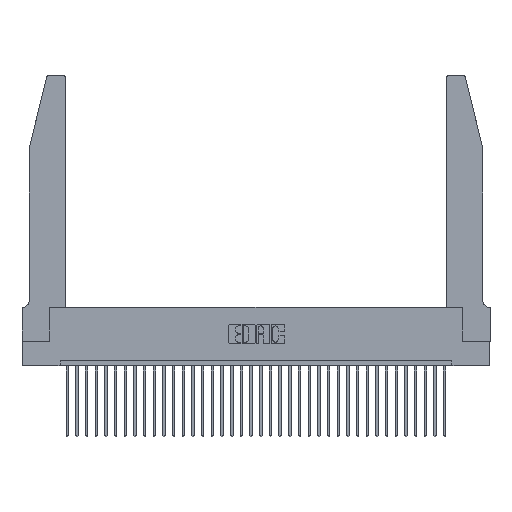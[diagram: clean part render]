
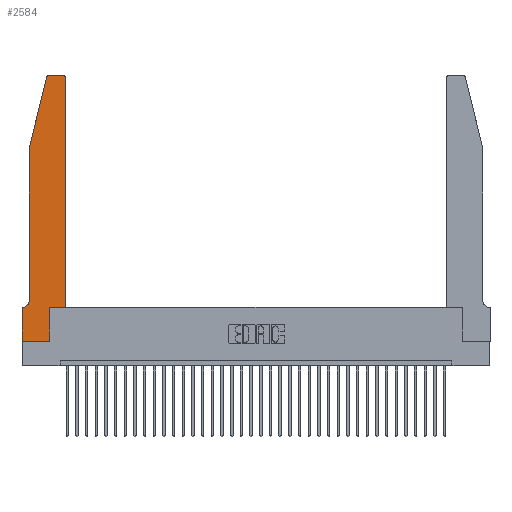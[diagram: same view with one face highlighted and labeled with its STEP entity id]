
A CAD part, top view. The second image highlights one B-rep face of the part: STEP entity #2584.
In plain terms, the highlighted planar face has unit normal (0, 0, 1).
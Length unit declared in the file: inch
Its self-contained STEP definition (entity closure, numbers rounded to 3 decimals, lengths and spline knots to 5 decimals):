
#125 = CIRCLE ( 'NONE', #30593, 0.03 ) ;
#261 = CARTESIAN_POINT ( 'NONE',  ( 0., 0., 0.37 ) ) ;
#321 = CARTESIAN_POINT ( 'NONE',  ( 0., 0.35, 0.37 ) ) ;
#1125 = DIRECTION ( 'NONE',  ( 1., 0., 0. ) ) ;
#1265 = VERTEX_POINT ( 'NONE', #3674 ) ;
#1301 = CARTESIAN_POINT ( 'NONE',  ( 0., 0.35, 0.37 ) ) ;
#1303 = CARTESIAN_POINT ( 'NONE',  ( 0.2605, 2.75, 0.37 ) ) ;
#1417 = LINE ( 'NONE', #9834, #13725 ) ;
#1427 = DIRECTION ( 'NONE',  ( 0., 0., 1. ) ) ;
#1449 = VECTOR ( 'NONE', #31238, 39.37008 ) ;
#1497 = EDGE_CURVE ( 'NONE', #5400, #5403, #125, .T. ) ;
#2011 = AXIS2_PLACEMENT_3D ( 'NONE', #25302, #30796, #19511 ) ;
#2113 = ORIENTED_EDGE ( 'NONE', *, *, #17704, .T. ) ;
#2464 = CARTESIAN_POINT ( 'NONE',  ( 0.4205, 2.75, 0.37 ) ) ;
#2584 = ADVANCED_FACE ( 'NONE', ( #22401 ), #12337, .T. ) ;
#3387 = LINE ( 'NONE', #6572, #30611 ) ;
#3674 = CARTESIAN_POINT ( 'NONE',  ( 0.0755, 0.42, 0.37 ) ) ;
#3752 = CARTESIAN_POINT ( 'NONE',  ( 0.2865, 0.35, 0.37 ) ) ;
#4170 = EDGE_CURVE ( 'NONE', #22668, #1265, #25288, .T. ) ;
#5089 = EDGE_CURVE ( 'NONE', #24419, #27045, #31650, .T. ) ;
#5400 = VERTEX_POINT ( 'NONE', #27581 ) ;
#5403 = VERTEX_POINT ( 'NONE', #19396 ) ;
#5968 = CIRCLE ( 'NONE', #24366, 0.03 ) ;
#6063 = CARTESIAN_POINT ( 'NONE',  ( 0.4505, 0.35, 0.37 ) ) ;
#6525 = LINE ( 'NONE', #1303, #1449 ) ;
#6572 = CARTESIAN_POINT ( 'NONE',  ( 0.2865, 0.35, 0.37 ) ) ;
#6644 = DIRECTION ( 'NONE',  ( 0., 0., 1. ) ) ;
#6650 = ORIENTED_EDGE ( 'NONE', *, *, #5089, .T. ) ;
#6679 = VERTEX_POINT ( 'NONE', #3752 ) ;
#7819 = DIRECTION ( 'NONE',  ( 0., -1., 0. ) ) ;
#8015 = CARTESIAN_POINT ( 'NONE',  ( 0.0755, 2., 0.37 ) ) ;
#8152 = ORIENTED_EDGE ( 'NONE', *, *, #4170, .T. ) ;
#8307 = CARTESIAN_POINT ( 'NONE',  ( 0.2865, 0., 0.37 ) ) ;
#8320 = CARTESIAN_POINT ( 'NONE',  ( 0.0755, 2., 0.37 ) ) ;
#8452 = CARTESIAN_POINT ( 'NONE',  ( 0.0755, 2., 0.37 ) ) ;
#8551 = DIRECTION ( 'NONE',  ( 0., -1., 0. ) ) ;
#9021 = AXIS2_PLACEMENT_3D ( 'NONE', #1301, #1427, #26003 ) ;
#9263 = VERTEX_POINT ( 'NONE', #25644 ) ;
#9834 = CARTESIAN_POINT ( 'NONE',  ( 0.0755, 0.35, 0.37 ) ) ;
#9888 = LINE ( 'NONE', #25170, #23463 ) ;
#10605 = EDGE_LOOP ( 'NONE', ( #25077, #29357, #11064, #8152, #22381, #32710, #6650, #26348, #23895, #2113, #23873, #28317 ) ) ;
#10652 = DIRECTION ( 'NONE',  ( -1., 0., 0. ) ) ;
#11064 = ORIENTED_EDGE ( 'NONE', *, *, #29533, .T. ) ;
#11788 = DIRECTION ( 'NONE',  ( 0., 1., 0. ) ) ;
#12337 = PLANE ( 'NONE',  #9021 ) ;
#12761 = VERTEX_POINT ( 'NONE', #15494 ) ;
#13193 = DIRECTION ( 'NONE',  ( 1., 0., 0. ) ) ;
#13408 = VERTEX_POINT ( 'NONE', #31011 ) ;
#13725 = VECTOR ( 'NONE', #10652, 39.37008 ) ;
#14202 = VECTOR ( 'NONE', #13193, 39.37008 ) ;
#14854 = DIRECTION ( 'NONE',  ( 1., 0., 0. ) ) ;
#15494 = CARTESIAN_POINT ( 'NONE',  ( 0.4505, 0.35, 0.37 ) ) ;
#16320 = EDGE_CURVE ( 'NONE', #27045, #30772, #27812, .T. ) ;
#16629 = EDGE_CURVE ( 'NONE', #24781, #5400, #6525, .T. ) ;
#16762 = EDGE_CURVE ( 'NONE', #13408, #24419, #1417, .T. ) ;
#17508 = DIRECTION ( 'NONE',  ( 0., 0., 1. ) ) ;
#17704 = EDGE_CURVE ( 'NONE', #6679, #12761, #9888, .T. ) ;
#17705 = LINE ( 'NONE', #8015, #34711 ) ;
#18554 = EDGE_CURVE ( 'NONE', #9263, #24781, #5968, .T. ) ;
#19069 = EDGE_CURVE ( 'NONE', #30772, #6679, #3387, .T. ) ;
#19089 = VECTOR ( 'NONE', #11788, 39.37008 ) ;
#19396 = CARTESIAN_POINT ( 'NONE',  ( 0.25487, 2.72718, 0.37 ) ) ;
#19511 = DIRECTION ( 'NONE',  ( -1., 0., 0. ) ) ;
#20169 = VECTOR ( 'NONE', #7819, 39.37008 ) ;
#22381 = ORIENTED_EDGE ( 'NONE', *, *, #33412, .T. ) ;
#22401 = FACE_OUTER_BOUND ( 'NONE', #10605, .T. ) ;
#22668 = VERTEX_POINT ( 'NONE', #8452 ) ;
#22935 = CARTESIAN_POINT ( 'NONE',  ( 0.4205, 2.72, 0.37 ) ) ;
#23463 = VECTOR ( 'NONE', #28424, 39.37008 ) ;
#23873 = ORIENTED_EDGE ( 'NONE', *, *, #33503, .T. ) ;
#23895 = ORIENTED_EDGE ( 'NONE', *, *, #19069, .T. ) ;
#24083 = CARTESIAN_POINT ( 'NONE',  ( 0., 0., 0.37 ) ) ;
#24366 = AXIS2_PLACEMENT_3D ( 'NONE', #22935, #6644, #14854 ) ;
#24419 = VERTEX_POINT ( 'NONE', #321 ) ;
#24781 = VERTEX_POINT ( 'NONE', #2464 ) ;
#25077 = ORIENTED_EDGE ( 'NONE', *, *, #16629, .T. ) ;
#25170 = CARTESIAN_POINT ( 'NONE',  ( 0.4505, 0.35, 0.37 ) ) ;
#25288 = LINE ( 'NONE', #8320, #28314 ) ;
#25302 = CARTESIAN_POINT ( 'NONE',  ( 0.0055, 0.42, 0.37 ) ) ;
#25644 = CARTESIAN_POINT ( 'NONE',  ( 0.4505, 2.72, 0.37 ) ) ;
#26003 = DIRECTION ( 'NONE',  ( 1., 0., 0. ) ) ;
#26348 = ORIENTED_EDGE ( 'NONE', *, *, #16320, .T. ) ;
#26755 = DIRECTION ( 'NONE',  ( -0.239, -0.971, 0. ) ) ;
#27045 = VERTEX_POINT ( 'NONE', #261 ) ;
#27581 = CARTESIAN_POINT ( 'NONE',  ( 0.284, 2.75, 0.37 ) ) ;
#27812 = LINE ( 'NONE', #31946, #14202 ) ;
#28314 = VECTOR ( 'NONE', #8551, 39.37008 ) ;
#28317 = ORIENTED_EDGE ( 'NONE', *, *, #18554, .T. ) ;
#28424 = DIRECTION ( 'NONE',  ( 1., 0., 0. ) ) ;
#28926 = LINE ( 'NONE', #6063, #19089 ) ;
#29343 = CIRCLE ( 'NONE', #2011, 0.07 ) ;
#29357 = ORIENTED_EDGE ( 'NONE', *, *, #1497, .T. ) ;
#29533 = EDGE_CURVE ( 'NONE', #5403, #22668, #17705, .T. ) ;
#30593 = AXIS2_PLACEMENT_3D ( 'NONE', #33676, #17508, #1125 ) ;
#30611 = VECTOR ( 'NONE', #31059, 39.37008 ) ;
#30772 = VERTEX_POINT ( 'NONE', #8307 ) ;
#30796 = DIRECTION ( 'NONE',  ( 0., 0., -1. ) ) ;
#31011 = CARTESIAN_POINT ( 'NONE',  ( 0.0055, 0.35, 0.37 ) ) ;
#31059 = DIRECTION ( 'NONE',  ( 0., 1., 0. ) ) ;
#31238 = DIRECTION ( 'NONE',  ( -1., 0., 0. ) ) ;
#31650 = LINE ( 'NONE', #24083, #20169 ) ;
#31946 = CARTESIAN_POINT ( 'NONE',  ( 0., 0., 0.37 ) ) ;
#32710 = ORIENTED_EDGE ( 'NONE', *, *, #16762, .T. ) ;
#33412 = EDGE_CURVE ( 'NONE', #1265, #13408, #29343, .T. ) ;
#33503 = EDGE_CURVE ( 'NONE', #12761, #9263, #28926, .T. ) ;
#33676 = CARTESIAN_POINT ( 'NONE',  ( 0.284, 2.72, 0.37 ) ) ;
#34711 = VECTOR ( 'NONE', #26755, 39.37008 ) ;
